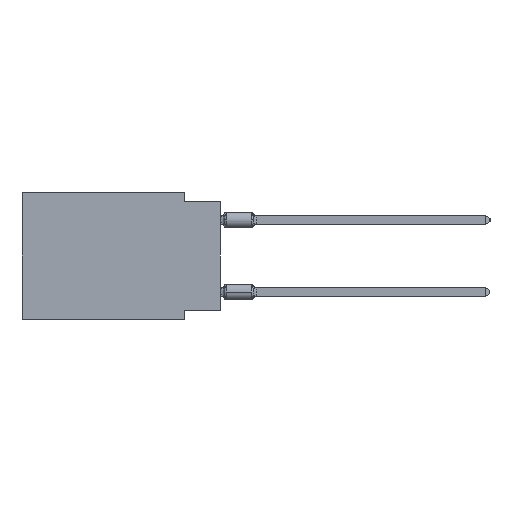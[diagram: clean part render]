
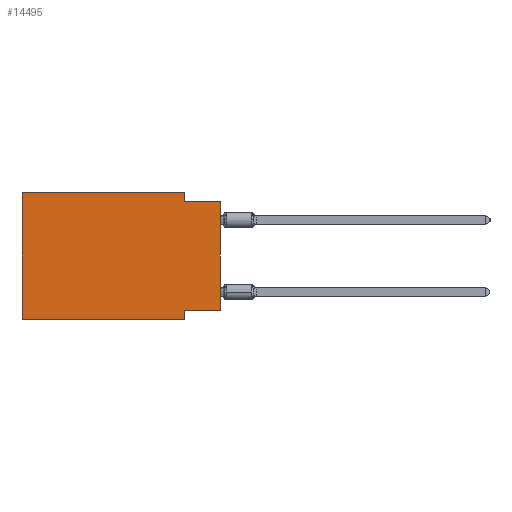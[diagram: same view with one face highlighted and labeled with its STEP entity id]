
A CAD part, left-side view. The second image highlights one B-rep face of the part: STEP entity #14495.
In plain terms, the highlighted planar face has unit normal (-1, 0, 0).
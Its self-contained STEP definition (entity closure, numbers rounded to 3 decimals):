
#661 = CARTESIAN_POINT ( 'NONE',  ( 0., 13.97, -8.89 ) ) ;
#832 = DIRECTION ( 'NONE',  ( 0., 1., 0. ) ) ;
#1133 = EDGE_CURVE ( 'NONE', #43026, #4743, #7175, .T. ) ;
#1751 = EDGE_LOOP ( 'NONE', ( #40109, #14039, #5051, #6507, #41182, #32073, #26666, #22633 ) ) ;
#3434 = DIRECTION ( 'NONE',  ( 0., 0., -1. ) ) ;
#4538 = LINE ( 'NONE', #11150, #11949 ) ;
#4743 = VERTEX_POINT ( 'NONE', #13465 ) ;
#5051 = ORIENTED_EDGE ( 'NONE', *, *, #36352, .F. ) ;
#6397 = LINE ( 'NONE', #30615, #23440 ) ;
#6507 = ORIENTED_EDGE ( 'NONE', *, *, #20467, .F. ) ;
#6832 = VERTEX_POINT ( 'NONE', #23857 ) ;
#7175 = LINE ( 'NONE', #38008, #11683 ) ;
#7458 = VERTEX_POINT ( 'NONE', #29913 ) ;
#7572 = VECTOR ( 'NONE', #31677, 1000. ) ;
#8419 = EDGE_CURVE ( 'NONE', #37390, #33168, #12089, .T. ) ;
#11150 = CARTESIAN_POINT ( 'NONE',  ( 0., 0., 0. ) ) ;
#11683 = VECTOR ( 'NONE', #24148, 1000. ) ;
#11949 = VECTOR ( 'NONE', #25031, 1000. ) ;
#12089 = LINE ( 'NONE', #12524, #24797 ) ;
#12524 = CARTESIAN_POINT ( 'NONE',  ( 0., 13.97, 0. ) ) ;
#13425 = CARTESIAN_POINT ( 'NONE',  ( 0., 0., -8.255 ) ) ;
#13465 = CARTESIAN_POINT ( 'NONE',  ( 0., 0., -0.635 ) ) ;
#13585 = LINE ( 'NONE', #27243, #21575 ) ;
#14039 = ORIENTED_EDGE ( 'NONE', *, *, #1133, .F. ) ;
#14495 = ADVANCED_FACE ( 'NONE', ( #38889 ), #19860, .F. ) ;
#16556 = DIRECTION ( 'NONE',  ( 1., 0., 0. ) ) ;
#17002 = VERTEX_POINT ( 'NONE', #40935 ) ;
#18238 = LINE ( 'NONE', #24212, #7572 ) ;
#19795 = DIRECTION ( 'NONE',  ( 0., 0., 1. ) ) ;
#19860 = PLANE ( 'NONE',  #27287 ) ;
#20467 = EDGE_CURVE ( 'NONE', #33168, #31200, #6397, .T. ) ;
#21575 = VECTOR ( 'NONE', #3434, 1000. ) ;
#22633 = ORIENTED_EDGE ( 'NONE', *, *, #29303, .F. ) ;
#23440 = VECTOR ( 'NONE', #30176, 1000. ) ;
#23857 = CARTESIAN_POINT ( 'NONE',  ( 0., 2.54, -8.255 ) ) ;
#24148 = DIRECTION ( 'NONE',  ( 0., -1., 0. ) ) ;
#24212 = CARTESIAN_POINT ( 'NONE',  ( 0., 13.97, -8.89 ) ) ;
#24797 = VECTOR ( 'NONE', #19795, 1000. ) ;
#25031 = DIRECTION ( 'NONE',  ( 0., 0., 1. ) ) ;
#25296 = CARTESIAN_POINT ( 'NONE',  ( 0., 2.54, -8.89 ) ) ;
#26666 = ORIENTED_EDGE ( 'NONE', *, *, #36296, .F. ) ;
#27243 = CARTESIAN_POINT ( 'NONE',  ( 0., 2.54, 0. ) ) ;
#27287 = AXIS2_PLACEMENT_3D ( 'NONE', #33313, #16556, #29982 ) ;
#29247 = LINE ( 'NONE', #25296, #37050 ) ;
#29303 = EDGE_CURVE ( 'NONE', #17002, #6832, #29305, .T. ) ;
#29305 = LINE ( 'NONE', #13425, #35183 ) ;
#29861 = EDGE_CURVE ( 'NONE', #17002, #4743, #4538, .T. ) ;
#29913 = CARTESIAN_POINT ( 'NONE',  ( 0., 2.54, -8.89 ) ) ;
#29982 = DIRECTION ( 'NONE',  ( 0., 0., -1. ) ) ;
#30176 = DIRECTION ( 'NONE',  ( 0., -1., 0. ) ) ;
#30615 = CARTESIAN_POINT ( 'NONE',  ( 0., 13.97, 0. ) ) ;
#31200 = VERTEX_POINT ( 'NONE', #34938 ) ;
#31677 = DIRECTION ( 'NONE',  ( 0., -1., 0. ) ) ;
#32005 = EDGE_CURVE ( 'NONE', #37390, #7458, #18238, .T. ) ;
#32073 = ORIENTED_EDGE ( 'NONE', *, *, #32005, .T. ) ;
#33168 = VERTEX_POINT ( 'NONE', #40936 ) ;
#33313 = CARTESIAN_POINT ( 'NONE',  ( 0., 13.97, 0. ) ) ;
#34077 = CARTESIAN_POINT ( 'NONE',  ( 0., 2.54, -0.635 ) ) ;
#34938 = CARTESIAN_POINT ( 'NONE',  ( 0., 2.54, 0. ) ) ;
#35183 = VECTOR ( 'NONE', #832, 1000. ) ;
#36296 = EDGE_CURVE ( 'NONE', #6832, #7458, #29247, .T. ) ;
#36352 = EDGE_CURVE ( 'NONE', #31200, #43026, #13585, .T. ) ;
#37050 = VECTOR ( 'NONE', #38960, 1000. ) ;
#37390 = VERTEX_POINT ( 'NONE', #661 ) ;
#38008 = CARTESIAN_POINT ( 'NONE',  ( 0., 0., -0.635 ) ) ;
#38889 = FACE_OUTER_BOUND ( 'NONE', #1751, .T. ) ;
#38960 = DIRECTION ( 'NONE',  ( 0., 0., -1. ) ) ;
#40109 = ORIENTED_EDGE ( 'NONE', *, *, #29861, .T. ) ;
#40935 = CARTESIAN_POINT ( 'NONE',  ( 0., 0., -8.255 ) ) ;
#40936 = CARTESIAN_POINT ( 'NONE',  ( 0., 13.97, 0. ) ) ;
#41182 = ORIENTED_EDGE ( 'NONE', *, *, #8419, .F. ) ;
#43026 = VERTEX_POINT ( 'NONE', #34077 ) ;
